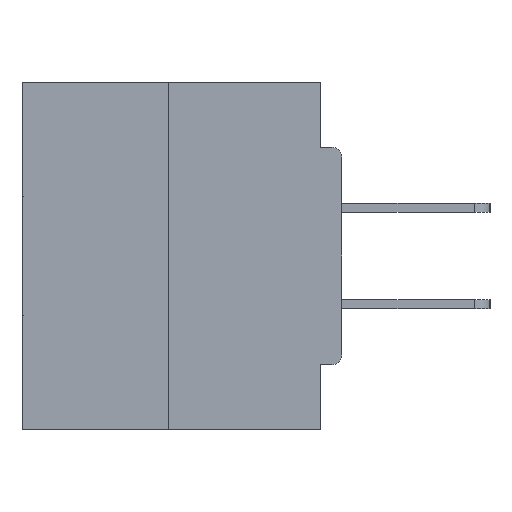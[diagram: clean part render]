
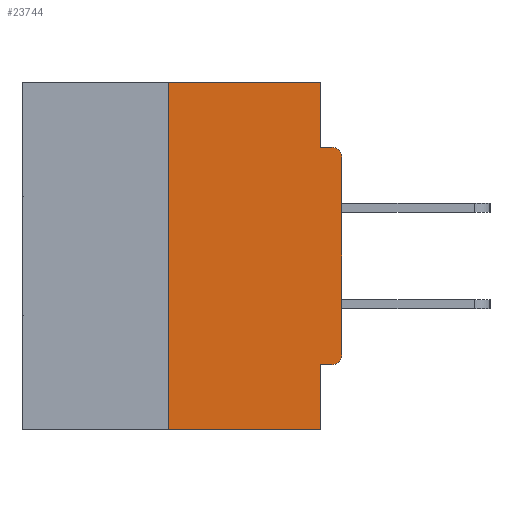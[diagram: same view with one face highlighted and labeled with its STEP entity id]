
A CAD part, left-side view. The second image highlights one B-rep face of the part: STEP entity #23744.
In plain terms, the highlighted planar face has unit normal (-1, 0, 0).
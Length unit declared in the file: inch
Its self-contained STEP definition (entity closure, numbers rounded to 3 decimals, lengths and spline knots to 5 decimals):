
#630 = CARTESIAN_POINT ( 'NONE',  ( 0., 0.031, -0.5 ) ) ;
#828 = VECTOR ( 'NONE', #1213, 39.37008 ) ;
#1213 = DIRECTION ( 'NONE',  ( 0., -1., 0. ) ) ;
#1399 = LINE ( 'NONE', #630, #39379 ) ;
#2294 = LINE ( 'NONE', #7408, #828 ) ;
#2744 = VECTOR ( 'NONE', #21739, 39.37008 ) ;
#3738 = DIRECTION ( 'NONE',  ( 0., 0., -1. ) ) ;
#4117 = CARTESIAN_POINT ( 'NONE',  ( 0., 0., -0.0935 ) ) ;
#4388 = VERTEX_POINT ( 'NONE', #18920 ) ;
#4922 = VECTOR ( 'NONE', #15654, 39.37008 ) ;
#5730 = EDGE_CURVE ( 'NONE', #39463, #32044, #27272, .T. ) ;
#5742 = VERTEX_POINT ( 'NONE', #28189 ) ;
#6358 = LINE ( 'NONE', #37446, #4922 ) ;
#6428 = DIRECTION ( 'NONE',  ( 1., 0., 0. ) ) ;
#7111 = DIRECTION ( 'NONE',  ( 0., 0., 1. ) ) ;
#7116 = VECTOR ( 'NONE', #13820, 39.37008 ) ;
#7148 = EDGE_CURVE ( 'NONE', #39347, #37571, #9326, .T. ) ;
#7408 = CARTESIAN_POINT ( 'NONE',  ( 0., 0.46, -0.5 ) ) ;
#7981 = EDGE_CURVE ( 'NONE', #32044, #16502, #6358, .T. ) ;
#8859 = AXIS2_PLACEMENT_3D ( 'NONE', #34840, #25692, #19618 ) ;
#9117 = PLANE ( 'NONE',  #38309 ) ;
#9326 = CIRCLE ( 'NONE', #8859, 0.015 ) ;
#9577 = DIRECTION ( 'NONE',  ( 0., 1., 0. ) ) ;
#9943 = ORIENTED_EDGE ( 'NONE', *, *, #36144, .F. ) ;
#10031 = ORIENTED_EDGE ( 'NONE', *, *, #20666, .T. ) ;
#10214 = EDGE_CURVE ( 'NONE', #5742, #39463, #33042, .T. ) ;
#10622 = AXIS2_PLACEMENT_3D ( 'NONE', #30180, #12003, #17510 ) ;
#10748 = CARTESIAN_POINT ( 'NONE',  ( 0., 0.25, 0. ) ) ;
#11047 = CARTESIAN_POINT ( 'NONE',  ( 0., 0.031, 0. ) ) ;
#11320 = CARTESIAN_POINT ( 'NONE',  ( 0., 0.25, 0. ) ) ;
#11840 = CARTESIAN_POINT ( 'NONE',  ( 0., 0.031, -0.0935 ) ) ;
#12003 = DIRECTION ( 'NONE',  ( -1., 0., 0. ) ) ;
#12178 = DIRECTION ( 'NONE',  ( 0., 0., -1. ) ) ;
#12747 = VECTOR ( 'NONE', #9577, 39.37008 ) ;
#12841 = EDGE_CURVE ( 'NONE', #31004, #28770, #1399, .T. ) ;
#13139 = CARTESIAN_POINT ( 'NONE',  ( 0., 0., 0. ) ) ;
#13476 = CARTESIAN_POINT ( 'NONE',  ( 0., 0.015, -0.4065 ) ) ;
#13820 = DIRECTION ( 'NONE',  ( 0., 0., 1. ) ) ;
#15522 = CARTESIAN_POINT ( 'NONE',  ( 0., 0.46, 0. ) ) ;
#15543 = ORIENTED_EDGE ( 'NONE', *, *, #12841, .F. ) ;
#15654 = DIRECTION ( 'NONE',  ( 0., 0., -1. ) ) ;
#16502 = VERTEX_POINT ( 'NONE', #11840 ) ;
#16565 = CIRCLE ( 'NONE', #10622, 0.015 ) ;
#16906 = LINE ( 'NONE', #13139, #25568 ) ;
#17268 = ORIENTED_EDGE ( 'NONE', *, *, #7981, .F. ) ;
#17510 = DIRECTION ( 'NONE',  ( 0., 0., -1. ) ) ;
#17667 = VERTEX_POINT ( 'NONE', #20292 ) ;
#18420 = EDGE_CURVE ( 'NONE', #16502, #17667, #19689, .T. ) ;
#18920 = CARTESIAN_POINT ( 'NONE',  ( 0., 0., -0.1085 ) ) ;
#19556 = ORIENTED_EDGE ( 'NONE', *, *, #18420, .F. ) ;
#19618 = DIRECTION ( 'NONE',  ( 0., 0., -1. ) ) ;
#19659 = DIRECTION ( 'NONE',  ( 0., -1., 0. ) ) ;
#19689 = LINE ( 'NONE', #4117, #34121 ) ;
#20292 = CARTESIAN_POINT ( 'NONE',  ( 0., 0.015, -0.0935 ) ) ;
#20666 = EDGE_CURVE ( 'NONE', #5742, #28770, #2294, .T. ) ;
#21739 = DIRECTION ( 'NONE',  ( 0., -1., 0. ) ) ;
#23744 = ADVANCED_FACE ( 'NONE', ( #32127 ), #9117, .F. ) ;
#24836 = EDGE_LOOP ( 'NONE', ( #33794, #38452, #10031, #15543, #9943, #38785, #36757, #28444, #19556, #17268 ) ) ;
#25568 = VECTOR ( 'NONE', #7111, 39.37008 ) ;
#25692 = DIRECTION ( 'NONE',  ( -1., 0., 0. ) ) ;
#25836 = EDGE_CURVE ( 'NONE', #4388, #17667, #16565, .T. ) ;
#27272 = LINE ( 'NONE', #28451, #2744 ) ;
#28189 = CARTESIAN_POINT ( 'NONE',  ( 0., 0.25, -0.5 ) ) ;
#28444 = ORIENTED_EDGE ( 'NONE', *, *, #25836, .T. ) ;
#28451 = CARTESIAN_POINT ( 'NONE',  ( 0., 0.46, 0. ) ) ;
#28770 = VERTEX_POINT ( 'NONE', #29930 ) ;
#29665 = CARTESIAN_POINT ( 'NONE',  ( 0., 0.031, -0.4065 ) ) ;
#29930 = CARTESIAN_POINT ( 'NONE',  ( 0., 0.031, -0.5 ) ) ;
#30180 = CARTESIAN_POINT ( 'NONE',  ( 0., 0.015, -0.1085 ) ) ;
#31004 = VERTEX_POINT ( 'NONE', #29665 ) ;
#31185 = CARTESIAN_POINT ( 'NONE',  ( 0., 0., -0.4065 ) ) ;
#31870 = EDGE_CURVE ( 'NONE', #37571, #4388, #16906, .T. ) ;
#32044 = VERTEX_POINT ( 'NONE', #11047 ) ;
#32127 = FACE_OUTER_BOUND ( 'NONE', #24836, .T. ) ;
#33042 = LINE ( 'NONE', #10748, #7116 ) ;
#33794 = ORIENTED_EDGE ( 'NONE', *, *, #5730, .F. ) ;
#34121 = VECTOR ( 'NONE', #19659, 39.37008 ) ;
#34840 = CARTESIAN_POINT ( 'NONE',  ( 0., 0.015, -0.3915 ) ) ;
#35661 = CARTESIAN_POINT ( 'NONE',  ( 0., 0., -0.3915 ) ) ;
#36144 = EDGE_CURVE ( 'NONE', #39347, #31004, #36310, .T. ) ;
#36310 = LINE ( 'NONE', #31185, #12747 ) ;
#36757 = ORIENTED_EDGE ( 'NONE', *, *, #31870, .T. ) ;
#37446 = CARTESIAN_POINT ( 'NONE',  ( 0., 0.031, 0. ) ) ;
#37571 = VERTEX_POINT ( 'NONE', #35661 ) ;
#38309 = AXIS2_PLACEMENT_3D ( 'NONE', #15522, #6428, #12178 ) ;
#38452 = ORIENTED_EDGE ( 'NONE', *, *, #10214, .F. ) ;
#38785 = ORIENTED_EDGE ( 'NONE', *, *, #7148, .T. ) ;
#39347 = VERTEX_POINT ( 'NONE', #13476 ) ;
#39379 = VECTOR ( 'NONE', #3738, 39.37008 ) ;
#39463 = VERTEX_POINT ( 'NONE', #11320 ) ;
